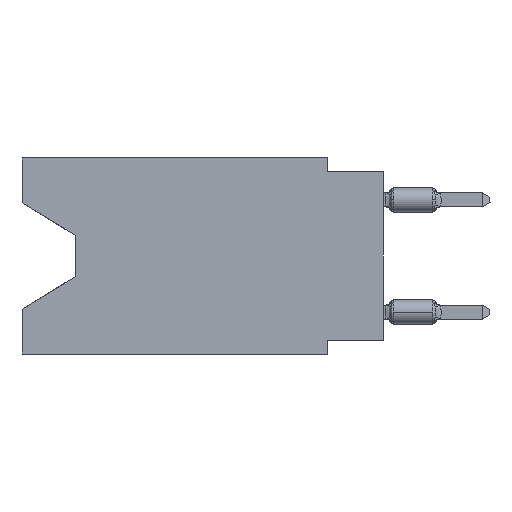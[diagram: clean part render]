
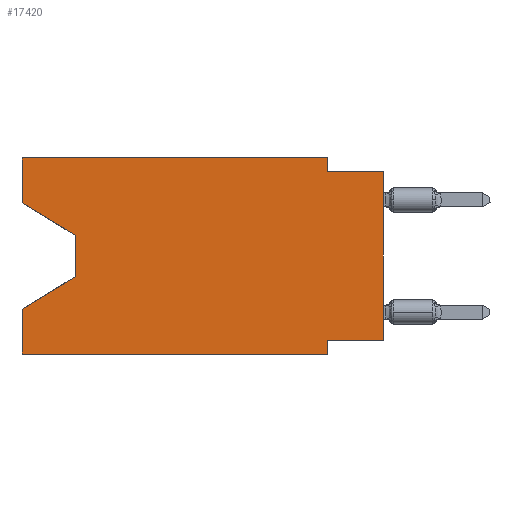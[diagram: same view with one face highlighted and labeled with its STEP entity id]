
A CAD part, left-side view. The second image highlights one B-rep face of the part: STEP entity #17420.
In plain terms, the highlighted planar face has unit normal (-1, 0, 0).
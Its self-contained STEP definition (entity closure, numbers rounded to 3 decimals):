
#1033 = CARTESIAN_POINT ( 'NONE',  ( 0., 0., -8.255 ) ) ;
#1212 = DIRECTION ( 'NONE',  ( 0., 0., 1. ) ) ;
#1769 = CARTESIAN_POINT ( 'NONE',  ( 0., 16.383, 0. ) ) ;
#1796 = CARTESIAN_POINT ( 'NONE',  ( 0., 2.54, -8.89 ) ) ;
#1888 = CARTESIAN_POINT ( 'NONE',  ( 0., 13.97, -3.505 ) ) ;
#2209 = LINE ( 'NONE', #1033, #17313 ) ;
#2515 = CARTESIAN_POINT ( 'NONE',  ( 0., 16.383, -8.89 ) ) ;
#2609 = ORIENTED_EDGE ( 'NONE', *, *, #42421, .T. ) ;
#3295 = CARTESIAN_POINT ( 'NONE',  ( 0., 2.54, 0. ) ) ;
#3814 = DIRECTION ( 'NONE',  ( 1., 0., 0. ) ) ;
#5441 = VECTOR ( 'NONE', #15269, 1000. ) ;
#5761 = DIRECTION ( 'NONE',  ( 0., 0., -1. ) ) ;
#6313 = ORIENTED_EDGE ( 'NONE', *, *, #25345, .T. ) ;
#7335 = VECTOR ( 'NONE', #58412, 1000. ) ;
#8250 = DIRECTION ( 'NONE',  ( 0., 0., 1. ) ) ;
#8361 = FACE_OUTER_BOUND ( 'NONE', #49115, .T. ) ;
#8730 = ORIENTED_EDGE ( 'NONE', *, *, #37805, .F. ) ;
#9602 = CARTESIAN_POINT ( 'NONE',  ( 0., 2.54, 0. ) ) ;
#9777 = ORIENTED_EDGE ( 'NONE', *, *, #24097, .F. ) ;
#11762 = CARTESIAN_POINT ( 'NONE',  ( 0., 2.54, -8.89 ) ) ;
#12169 = VERTEX_POINT ( 'NONE', #38557 ) ;
#13077 = EDGE_CURVE ( 'NONE', #15130, #18310, #26813, .T. ) ;
#13157 = ORIENTED_EDGE ( 'NONE', *, *, #42792, .F. ) ;
#14328 = DIRECTION ( 'NONE',  ( 0., 0.855, -0.519 ) ) ;
#15130 = VERTEX_POINT ( 'NONE', #32098 ) ;
#15269 = DIRECTION ( 'NONE',  ( 0., -1., 0. ) ) ;
#16444 = VERTEX_POINT ( 'NONE', #45374 ) ;
#17313 = VECTOR ( 'NONE', #20667, 1000. ) ;
#17420 = ADVANCED_FACE ( 'NONE', ( #8361 ), #26804, .F. ) ;
#17507 = VECTOR ( 'NONE', #54343, 1000. ) ;
#17794 = CARTESIAN_POINT ( 'NONE',  ( 0., 2.54, -8.255 ) ) ;
#18310 = VERTEX_POINT ( 'NONE', #56331 ) ;
#18423 = ORIENTED_EDGE ( 'NONE', *, *, #29582, .T. ) ;
#18440 = ORIENTED_EDGE ( 'NONE', *, *, #13077, .F. ) ;
#18606 = CARTESIAN_POINT ( 'NONE',  ( 0., 16.383, -6.852 ) ) ;
#18946 = ORIENTED_EDGE ( 'NONE', *, *, #33217, .T. ) ;
#19215 = EDGE_CURVE ( 'NONE', #12169, #49304, #44582, .T. ) ;
#19218 = LINE ( 'NONE', #43071, #5441 ) ;
#20242 = LINE ( 'NONE', #1769, #56879 ) ;
#20667 = DIRECTION ( 'NONE',  ( 0., 1., 0. ) ) ;
#20897 = VERTEX_POINT ( 'NONE', #2515 ) ;
#21301 = CARTESIAN_POINT ( 'NONE',  ( 0., 16.383, -2.038 ) ) ;
#21362 = CARTESIAN_POINT ( 'NONE',  ( 0., 16.383, -8.89 ) ) ;
#21571 = CARTESIAN_POINT ( 'NONE',  ( 0., 0., 0. ) ) ;
#21823 = LINE ( 'NONE', #53290, #7335 ) ;
#21949 = LINE ( 'NONE', #21362, #27660 ) ;
#22460 = VERTEX_POINT ( 'NONE', #45498 ) ;
#23783 = ORIENTED_EDGE ( 'NONE', *, *, #28719, .F. ) ;
#24097 = EDGE_CURVE ( 'NONE', #16444, #29911, #2209, .T. ) ;
#25345 = EDGE_CURVE ( 'NONE', #16444, #18310, #48763, .T. ) ;
#25580 = DIRECTION ( 'NONE',  ( 0., -1., 0. ) ) ;
#26136 = AXIS2_PLACEMENT_3D ( 'NONE', #45240, #3814, #40729 ) ;
#26804 = PLANE ( 'NONE',  #26136 ) ;
#26813 = LINE ( 'NONE', #48874, #17507 ) ;
#27660 = VECTOR ( 'NONE', #25580, 1000. ) ;
#28564 = EDGE_CURVE ( 'NONE', #29911, #41951, #34173, .T. ) ;
#28667 = VERTEX_POINT ( 'NONE', #3295 ) ;
#28719 = EDGE_CURVE ( 'NONE', #20897, #48117, #53195, .T. ) ;
#29582 = EDGE_CURVE ( 'NONE', #49304, #22460, #21823, .T. ) ;
#29911 = VERTEX_POINT ( 'NONE', #17794 ) ;
#30368 = DIRECTION ( 'NONE',  ( 0., -0.855, -0.519 ) ) ;
#31188 = ORIENTED_EDGE ( 'NONE', *, *, #28564, .F. ) ;
#32098 = CARTESIAN_POINT ( 'NONE',  ( 0., 2.54, -0.635 ) ) ;
#33191 = DIRECTION ( 'NONE',  ( 0., 0., -1. ) ) ;
#33217 = EDGE_CURVE ( 'NONE', #22460, #48117, #40646, .T. ) ;
#34173 = LINE ( 'NONE', #1796, #58423 ) ;
#36689 = VECTOR ( 'NONE', #8250, 1000. ) ;
#37575 = EDGE_CURVE ( 'NONE', #28667, #15130, #42258, .T. ) ;
#37805 = EDGE_CURVE ( 'NONE', #12169, #57012, #20242, .T. ) ;
#38498 = VECTOR ( 'NONE', #33191, 1000. ) ;
#38557 = CARTESIAN_POINT ( 'NONE',  ( 0., 16.383, -2.038 ) ) ;
#39007 = CARTESIAN_POINT ( 'NONE',  ( 0., 16.383, 0. ) ) ;
#39903 = DIRECTION ( 'NONE',  ( 0., 0., 1. ) ) ;
#40083 = VECTOR ( 'NONE', #39903, 1000. ) ;
#40646 = LINE ( 'NONE', #59094, #50788 ) ;
#40729 = DIRECTION ( 'NONE',  ( 0., 0., -1. ) ) ;
#41951 = VERTEX_POINT ( 'NONE', #11762 ) ;
#42258 = LINE ( 'NONE', #9602, #38498 ) ;
#42421 = EDGE_CURVE ( 'NONE', #20897, #41951, #21949, .T. ) ;
#42792 = EDGE_CURVE ( 'NONE', #57012, #28667, #19218, .T. ) ;
#43071 = CARTESIAN_POINT ( 'NONE',  ( 0., 16.383, 0. ) ) ;
#44278 = ORIENTED_EDGE ( 'NONE', *, *, #37575, .F. ) ;
#44582 = LINE ( 'NONE', #21301, #46521 ) ;
#45240 = CARTESIAN_POINT ( 'NONE',  ( 0., 16.383, 0. ) ) ;
#45374 = CARTESIAN_POINT ( 'NONE',  ( 0., 0., -8.255 ) ) ;
#45498 = CARTESIAN_POINT ( 'NONE',  ( 0., 13.97, -5.385 ) ) ;
#46521 = VECTOR ( 'NONE', #30368, 1000. ) ;
#48117 = VERTEX_POINT ( 'NONE', #18606 ) ;
#48763 = LINE ( 'NONE', #21571, #36689 ) ;
#48874 = CARTESIAN_POINT ( 'NONE',  ( 0., 0., -0.635 ) ) ;
#49115 = EDGE_LOOP ( 'NONE', ( #52633, #18423, #18946, #23783, #2609, #31188, #9777, #6313, #18440, #44278, #13157, #8730 ) ) ;
#49304 = VERTEX_POINT ( 'NONE', #1888 ) ;
#50788 = VECTOR ( 'NONE', #14328, 1000. ) ;
#52633 = ORIENTED_EDGE ( 'NONE', *, *, #19215, .T. ) ;
#53195 = LINE ( 'NONE', #39007, #40083 ) ;
#53290 = CARTESIAN_POINT ( 'NONE',  ( 0., 13.97, -3.505 ) ) ;
#54343 = DIRECTION ( 'NONE',  ( 0., -1., 0. ) ) ;
#56331 = CARTESIAN_POINT ( 'NONE',  ( 0., 0., -0.635 ) ) ;
#56879 = VECTOR ( 'NONE', #1212, 1000. ) ;
#57012 = VERTEX_POINT ( 'NONE', #59088 ) ;
#58412 = DIRECTION ( 'NONE',  ( 0., 0., -1. ) ) ;
#58423 = VECTOR ( 'NONE', #5761, 1000. ) ;
#59088 = CARTESIAN_POINT ( 'NONE',  ( 0., 16.383, 0. ) ) ;
#59094 = CARTESIAN_POINT ( 'NONE',  ( 0., 13.97, -5.385 ) ) ;
